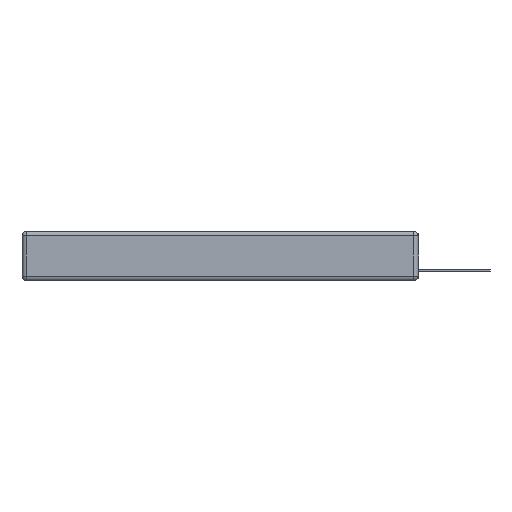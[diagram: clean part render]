
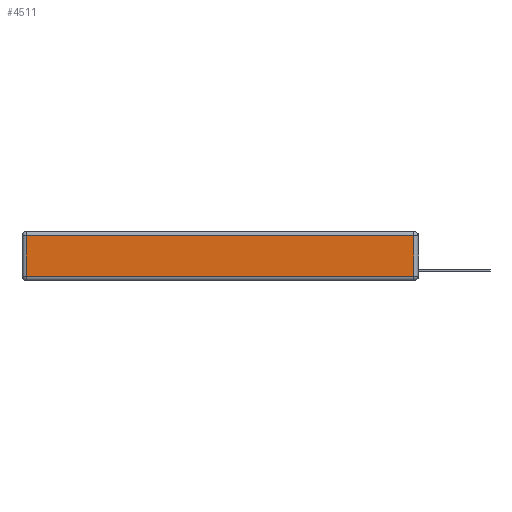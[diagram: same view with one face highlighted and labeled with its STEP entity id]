
A CAD part, left-side view. The second image highlights one B-rep face of the part: STEP entity #4511.
In plain terms, the highlighted planar face has unit normal (-1, 0, 0).
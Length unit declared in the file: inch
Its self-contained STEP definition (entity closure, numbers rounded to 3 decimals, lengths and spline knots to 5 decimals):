
#324 = EDGE_CURVE ( 'NONE', #1784, #14865, #14684, .T. ) ;
#441 = CARTESIAN_POINT ( 'NONE',  ( 0., 2.72, -0.03 ) ) ;
#1319 = AXIS2_PLACEMENT_3D ( 'NONE', #16395, #2805, #5513 ) ;
#1784 = VERTEX_POINT ( 'NONE', #441 ) ;
#1843 = ORIENTED_EDGE ( 'NONE', *, *, #4195, .T. ) ;
#2805 = DIRECTION ( 'NONE',  ( -1., 0., 0. ) ) ;
#3248 = LINE ( 'NONE', #15769, #13150 ) ;
#4195 = EDGE_CURVE ( 'NONE', #9639, #1784, #3248, .T. ) ;
#4511 = ADVANCED_FACE ( 'NONE', ( #16934 ), #5616, .T. ) ;
#4559 = DIRECTION ( 'NONE',  ( 0., 0., 1. ) ) ;
#5010 = EDGE_LOOP ( 'NONE', ( #12580, #5947, #1843, #13529 ) ) ;
#5513 = DIRECTION ( 'NONE',  ( 0., 0., 1. ) ) ;
#5616 = PLANE ( 'NONE',  #1319 ) ;
#5759 = CARTESIAN_POINT ( 'NONE',  ( 0., 0.03, -0.03 ) ) ;
#5947 = ORIENTED_EDGE ( 'NONE', *, *, #10844, .T. ) ;
#6286 = CARTESIAN_POINT ( 'NONE',  ( 0., 2.72, -0.343 ) ) ;
#7913 = VECTOR ( 'NONE', #4559, 39.37008 ) ;
#8487 = DIRECTION ( 'NONE',  ( 0., -1., 0. ) ) ;
#9017 = DIRECTION ( 'NONE',  ( 0., 1., 0. ) ) ;
#9639 = VERTEX_POINT ( 'NONE', #5759 ) ;
#10056 = CARTESIAN_POINT ( 'NONE',  ( 0., 0.03, -0.343 ) ) ;
#10190 = EDGE_CURVE ( 'NONE', #14865, #12312, #12577, .T. ) ;
#10844 = EDGE_CURVE ( 'NONE', #12312, #9639, #12768, .T. ) ;
#11292 = VECTOR ( 'NONE', #8487, 39.37008 ) ;
#11638 = DIRECTION ( 'NONE',  ( 0., 0., -1. ) ) ;
#12312 = VERTEX_POINT ( 'NONE', #15997 ) ;
#12577 = LINE ( 'NONE', #15043, #11292 ) ;
#12580 = ORIENTED_EDGE ( 'NONE', *, *, #10190, .T. ) ;
#12768 = LINE ( 'NONE', #10056, #7913 ) ;
#13150 = VECTOR ( 'NONE', #9017, 39.37008 ) ;
#13529 = ORIENTED_EDGE ( 'NONE', *, *, #324, .T. ) ;
#14275 = VECTOR ( 'NONE', #11638, 39.37008 ) ;
#14684 = LINE ( 'NONE', #6286, #14275 ) ;
#14865 = VERTEX_POINT ( 'NONE', #16750 ) ;
#15043 = CARTESIAN_POINT ( 'NONE',  ( 0., 0., -0.313 ) ) ;
#15769 = CARTESIAN_POINT ( 'NONE',  ( 0., 2.75, -0.03 ) ) ;
#15997 = CARTESIAN_POINT ( 'NONE',  ( 0., 0.03, -0.313 ) ) ;
#16395 = CARTESIAN_POINT ( 'NONE',  ( 0., 0., -0.343 ) ) ;
#16750 = CARTESIAN_POINT ( 'NONE',  ( 0., 2.72, -0.313 ) ) ;
#16934 = FACE_OUTER_BOUND ( 'NONE', #5010, .T. ) ;
